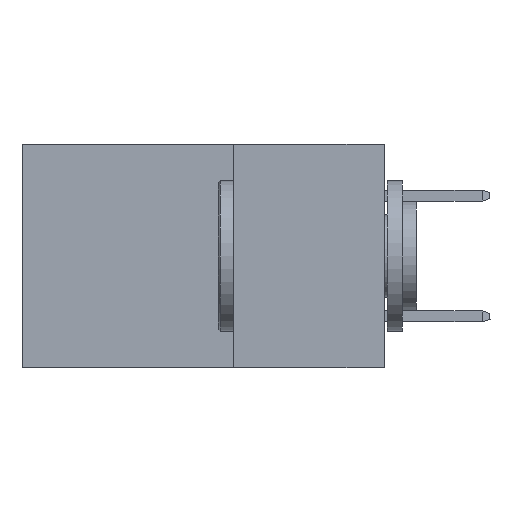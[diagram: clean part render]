
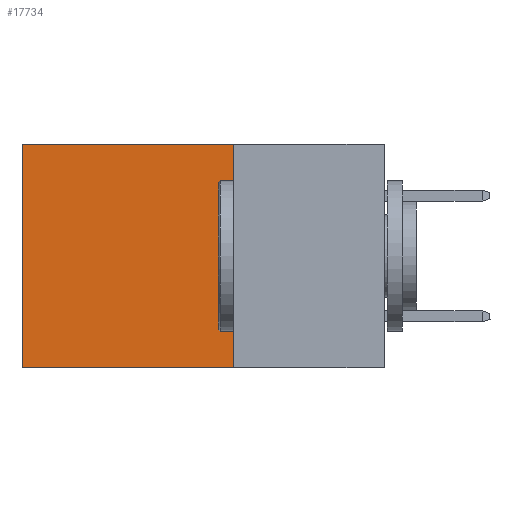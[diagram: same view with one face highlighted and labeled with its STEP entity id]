
A CAD part, left-side view. The second image highlights one B-rep face of the part: STEP entity #17734.
In plain terms, the highlighted planar face has unit normal (-1, 0, 0).
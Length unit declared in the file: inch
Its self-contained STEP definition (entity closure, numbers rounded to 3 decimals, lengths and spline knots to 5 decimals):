
#465 = CARTESIAN_POINT ( 'NONE',  ( 0.2615, 0.25, 0. ) ) ;
#738 = FACE_OUTER_BOUND ( 'NONE', #9200, .T. ) ;
#2383 = VECTOR ( 'NONE', #18185, 39.37008 ) ;
#3050 = LINE ( 'NONE', #6000, #2383 ) ;
#3074 = ORIENTED_EDGE ( 'NONE', *, *, #25572, .F. ) ;
#3618 = CARTESIAN_POINT ( 'NONE',  ( 0.2615, 0.25, -0.37 ) ) ;
#4584 = AXIS2_PLACEMENT_3D ( 'NONE', #16974, #4722, #18973 ) ;
#4722 = DIRECTION ( 'NONE',  ( 1., 0., 0. ) ) ;
#5651 = DIRECTION ( 'NONE',  ( 0., 0., -1. ) ) ;
#5676 = CARTESIAN_POINT ( 'NONE',  ( 0.2615, 0.6, 0. ) ) ;
#6000 = CARTESIAN_POINT ( 'NONE',  ( 0.2615, 0.25, -0.37 ) ) ;
#6170 = LINE ( 'NONE', #465, #21674 ) ;
#6733 = LINE ( 'NONE', #15850, #11570 ) ;
#6950 = LINE ( 'NONE', #18888, #17149 ) ;
#7565 = VERTEX_POINT ( 'NONE', #3618 ) ;
#7834 = VERTEX_POINT ( 'NONE', #8067 ) ;
#8067 = CARTESIAN_POINT ( 'NONE',  ( 0.2615, 0.6, -0.37 ) ) ;
#9200 = EDGE_LOOP ( 'NONE', ( #9400, #12057, #3074, #18180 ) ) ;
#9400 = ORIENTED_EDGE ( 'NONE', *, *, #23211, .T. ) ;
#10398 = CARTESIAN_POINT ( 'NONE',  ( 0.2615, 0.25, 0. ) ) ;
#10887 = PLANE ( 'NONE',  #4584 ) ;
#11570 = VECTOR ( 'NONE', #5651, 39.37008 ) ;
#12057 = ORIENTED_EDGE ( 'NONE', *, *, #17731, .F. ) ;
#12780 = VERTEX_POINT ( 'NONE', #5676 ) ;
#15850 = CARTESIAN_POINT ( 'NONE',  ( 0.2615, 0.6, -0.37 ) ) ;
#16974 = CARTESIAN_POINT ( 'NONE',  ( 0.2615, 0.25, -0.37 ) ) ;
#17149 = VECTOR ( 'NONE', #24835, 39.37008 ) ;
#17731 = EDGE_CURVE ( 'NONE', #7565, #7834, #6950, .T. ) ;
#17734 = ADVANCED_FACE ( 'NONE', ( #738 ), #10887, .F. ) ;
#18180 = ORIENTED_EDGE ( 'NONE', *, *, #21064, .T. ) ;
#18185 = DIRECTION ( 'NONE',  ( 0., 0., -1. ) ) ;
#18888 = CARTESIAN_POINT ( 'NONE',  ( 0.2615, 0.25, -0.37 ) ) ;
#18973 = DIRECTION ( 'NONE',  ( 0., 0., -1. ) ) ;
#21064 = EDGE_CURVE ( 'NONE', #22149, #12780, #6170, .T. ) ;
#21674 = VECTOR ( 'NONE', #22856, 39.37008 ) ;
#22149 = VERTEX_POINT ( 'NONE', #10398 ) ;
#22856 = DIRECTION ( 'NONE',  ( 0., 1., 0. ) ) ;
#23211 = EDGE_CURVE ( 'NONE', #12780, #7834, #6733, .T. ) ;
#24835 = DIRECTION ( 'NONE',  ( 0., 1., 0. ) ) ;
#25572 = EDGE_CURVE ( 'NONE', #22149, #7565, #3050, .T. ) ;
